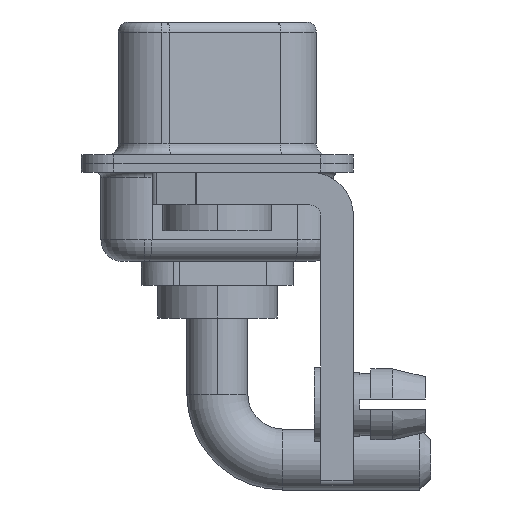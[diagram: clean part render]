
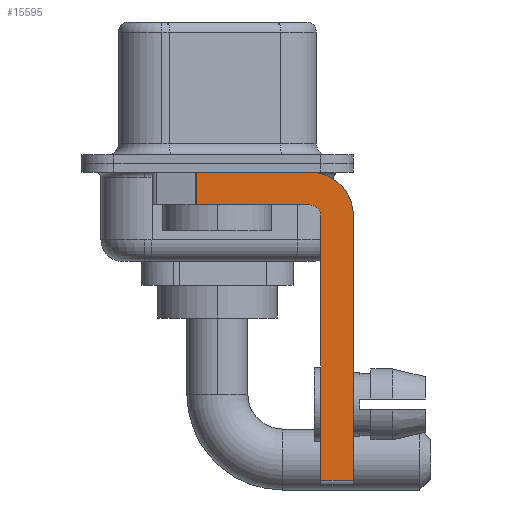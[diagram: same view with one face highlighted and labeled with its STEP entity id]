
A CAD part, left-side view. The second image highlights one B-rep face of the part: STEP entity #15595.
In plain terms, the highlighted planar face has unit normal (-1, 0, 0).
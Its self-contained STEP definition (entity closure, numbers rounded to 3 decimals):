
#67 = VERTEX_POINT ( 'NONE', #7644 ) ;
#183 = CARTESIAN_POINT ( 'NONE',  ( -2.9, -6.25, -14.55 ) ) ;
#423 = CARTESIAN_POINT ( 'NONE',  ( -2.9, -6.25, -2.4 ) ) ;
#584 = LINE ( 'NONE', #7647, #16981 ) ;
#585 = EDGE_CURVE ( 'NONE', #11409, #6674, #584, .T. ) ;
#757 = LINE ( 'NONE', #16607, #17119 ) ;
#1315 = AXIS2_PLACEMENT_3D ( 'NONE', #2062, #14999, #6486 ) ;
#1866 = VERTEX_POINT ( 'NONE', #12193 ) ;
#2049 = DIRECTION ( 'NONE',  ( 0., 1., 0. ) ) ;
#2057 = DIRECTION ( 'NONE',  ( 0., 0., -1. ) ) ;
#2062 = CARTESIAN_POINT ( 'NONE',  ( -2.9, -4.25, -2.4 ) ) ;
#2131 = ORIENTED_EDGE ( 'NONE', *, *, #16601, .F. ) ;
#2165 = CARTESIAN_POINT ( 'NONE',  ( -2.9, -4.75, -2.4 ) ) ;
#2269 = ORIENTED_EDGE ( 'NONE', *, *, #5876, .F. ) ;
#2597 = CARTESIAN_POINT ( 'NONE',  ( -2.9, 3., -0.4 ) ) ;
#2653 = VECTOR ( 'NONE', #2049, 1000. ) ;
#2657 = ORIENTED_EDGE ( 'NONE', *, *, #11040, .F. ) ;
#3084 = EDGE_LOOP ( 'NONE', ( #2131, #5819, #11182, #2269, #8467, #15862, #11779, #2657 ) ) ;
#3535 = CARTESIAN_POINT ( 'NONE',  ( -2.9, -4.25, -0.4 ) ) ;
#3732 = CARTESIAN_POINT ( 'NONE',  ( -2.9, -4.25, -1.9 ) ) ;
#3748 = FACE_OUTER_BOUND ( 'NONE', #3084, .T. ) ;
#4191 = LINE ( 'NONE', #2597, #10698 ) ;
#4312 = DIRECTION ( 'NONE',  ( 0., -1., 0. ) ) ;
#5615 = CARTESIAN_POINT ( 'NONE',  ( -2.9, -4.25, -2.4 ) ) ;
#5754 = EDGE_CURVE ( 'NONE', #1866, #67, #9476, .T. ) ;
#5819 = ORIENTED_EDGE ( 'NONE', *, *, #17050, .T. ) ;
#5876 = EDGE_CURVE ( 'NONE', #8189, #1866, #13200, .T. ) ;
#5889 = VECTOR ( 'NONE', #16910, 1000. ) ;
#5931 = DIRECTION ( 'NONE',  ( 1., 0., 0. ) ) ;
#6052 = CARTESIAN_POINT ( 'NONE',  ( -2.9, 0.978, -0.4 ) ) ;
#6474 = EDGE_CURVE ( 'NONE', #14074, #8189, #757, .T. ) ;
#6486 = DIRECTION ( 'NONE',  ( 0., 0., -1. ) ) ;
#6508 = DIRECTION ( 'NONE',  ( 0., 0., 1. ) ) ;
#6674 = VERTEX_POINT ( 'NONE', #183 ) ;
#6814 = CARTESIAN_POINT ( 'NONE',  ( -2.9, 0.978, -1.9 ) ) ;
#7081 = EDGE_CURVE ( 'NONE', #14074, #6674, #17142, .T. ) ;
#7644 = CARTESIAN_POINT ( 'NONE',  ( -2.9, 0.978, -1.9 ) ) ;
#7647 = CARTESIAN_POINT ( 'NONE',  ( -2.9, -6.25, -2.4 ) ) ;
#8189 = VERTEX_POINT ( 'NONE', #2165 ) ;
#8363 = AXIS2_PLACEMENT_3D ( 'NONE', #5615, #15429, #11375 ) ;
#8385 = VECTOR ( 'NONE', #4312, 1000. ) ;
#8467 = ORIENTED_EDGE ( 'NONE', *, *, #6474, .F. ) ;
#9476 = LINE ( 'NONE', #3732, #2653 ) ;
#10344 = CARTESIAN_POINT ( 'NONE',  ( -2.9, -4.25, -2.4 ) ) ;
#10698 = VECTOR ( 'NONE', #11372, 1000. ) ;
#10741 = PLANE ( 'NONE',  #1315 ) ;
#11040 = EDGE_CURVE ( 'NONE', #17032, #11409, #13336, .T. ) ;
#11182 = ORIENTED_EDGE ( 'NONE', *, *, #5754, .F. ) ;
#11372 = DIRECTION ( 'NONE',  ( 0., -1., 0. ) ) ;
#11375 = DIRECTION ( 'NONE',  ( 0., 0., 1. ) ) ;
#11409 = VERTEX_POINT ( 'NONE', #423 ) ;
#11779 = ORIENTED_EDGE ( 'NONE', *, *, #585, .F. ) ;
#12193 = CARTESIAN_POINT ( 'NONE',  ( -2.9, -4.25, -1.9 ) ) ;
#12437 = AXIS2_PLACEMENT_3D ( 'NONE', #10344, #5931, #2057 ) ;
#12554 = CARTESIAN_POINT ( 'NONE',  ( -2.9, -4.75, -14.55 ) ) ;
#13200 = CIRCLE ( 'NONE', #8363, 0.5 ) ;
#13336 = CIRCLE ( 'NONE', #12437, 2. ) ;
#13414 = DIRECTION ( 'NONE',  ( 0., 0., -1. ) ) ;
#14074 = VERTEX_POINT ( 'NONE', #12554 ) ;
#14705 = CARTESIAN_POINT ( 'NONE',  ( -2.9, -4.25, -14.55 ) ) ;
#14999 = DIRECTION ( 'NONE',  ( 1., 0., 0. ) ) ;
#15429 = DIRECTION ( 'NONE',  ( -1., 0., 0. ) ) ;
#15595 = ADVANCED_FACE ( 'NONE', ( #3748 ), #10741, .F. ) ;
#15862 = ORIENTED_EDGE ( 'NONE', *, *, #7081, .T. ) ;
#16242 = VERTEX_POINT ( 'NONE', #6052 ) ;
#16601 = EDGE_CURVE ( 'NONE', #16242, #17032, #4191, .T. ) ;
#16607 = CARTESIAN_POINT ( 'NONE',  ( -2.9, -4.75, -14.8 ) ) ;
#16728 = LINE ( 'NONE', #6814, #5889 ) ;
#16910 = DIRECTION ( 'NONE',  ( 0., 0., -1. ) ) ;
#16981 = VECTOR ( 'NONE', #13414, 1000. ) ;
#17032 = VERTEX_POINT ( 'NONE', #3535 ) ;
#17050 = EDGE_CURVE ( 'NONE', #16242, #67, #16728, .T. ) ;
#17119 = VECTOR ( 'NONE', #6508, 1000. ) ;
#17142 = LINE ( 'NONE', #14705, #8385 ) ;
